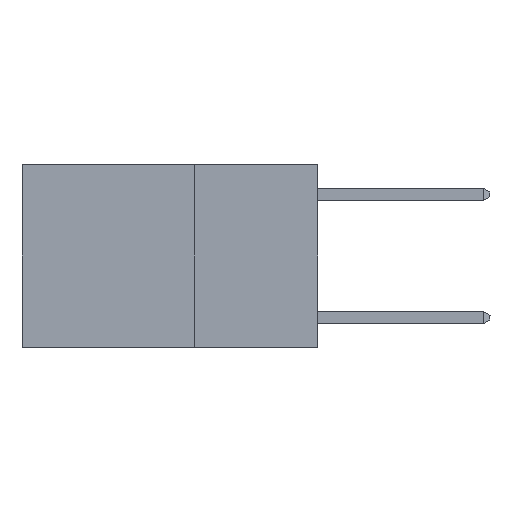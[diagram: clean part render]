
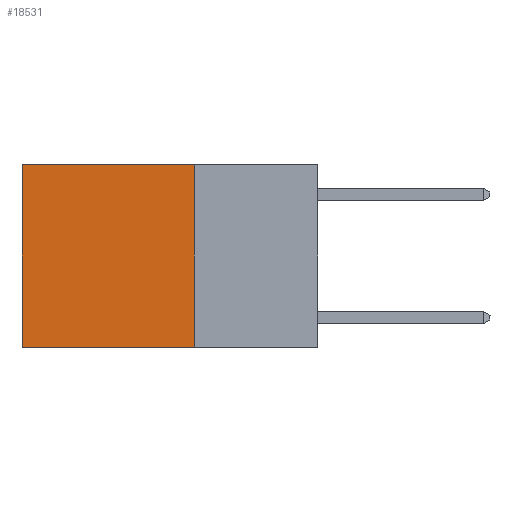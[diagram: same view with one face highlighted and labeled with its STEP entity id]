
A CAD part, left-side view. The second image highlights one B-rep face of the part: STEP entity #18531.
In plain terms, the highlighted planar face has unit normal (-1, 0, 0).
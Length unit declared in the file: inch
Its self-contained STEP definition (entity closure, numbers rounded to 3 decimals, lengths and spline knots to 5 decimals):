
#1092 = DIRECTION ( 'NONE',  ( 0., 0., -1. ) ) ;
#1262 = DIRECTION ( 'NONE',  ( 1., 0., 0. ) ) ;
#1551 = VECTOR ( 'NONE', #5936, 39.37008 ) ;
#1714 = VECTOR ( 'NONE', #1092, 39.37008 ) ;
#1950 = CARTESIAN_POINT ( 'NONE',  ( 0.2625, 0.25, 0. ) ) ;
#2614 = VERTEX_POINT ( 'NONE', #6307 ) ;
#3176 = EDGE_CURVE ( 'NONE', #8763, #2614, #7273, .T. ) ;
#3692 = VECTOR ( 'NONE', #7816, 39.37008 ) ;
#4391 = CARTESIAN_POINT ( 'NONE',  ( 0.2625, 0.25, -0.37 ) ) ;
#5743 = LINE ( 'NONE', #7167, #1714 ) ;
#5936 = DIRECTION ( 'NONE',  ( 0., 0., -1. ) ) ;
#6307 = CARTESIAN_POINT ( 'NONE',  ( 0.2625, 0.6, -0.37 ) ) ;
#7167 = CARTESIAN_POINT ( 'NONE',  ( 0.2625, 0.25, 0. ) ) ;
#7273 = LINE ( 'NONE', #18326, #3692 ) ;
#7395 = CARTESIAN_POINT ( 'NONE',  ( 0.2625, 0.6, 0. ) ) ;
#7660 = EDGE_CURVE ( 'NONE', #11700, #14391, #18274, .T. ) ;
#7816 = DIRECTION ( 'NONE',  ( 0., 1., 0. ) ) ;
#8507 = VECTOR ( 'NONE', #9395, 39.37008 ) ;
#8763 = VERTEX_POINT ( 'NONE', #4391 ) ;
#9139 = LINE ( 'NONE', #19642, #1551 ) ;
#9267 = CARTESIAN_POINT ( 'NONE',  ( 0.2625, 0.25, 0. ) ) ;
#9395 = DIRECTION ( 'NONE',  ( 0., 1., 0. ) ) ;
#11389 = ORIENTED_EDGE ( 'NONE', *, *, #15072, .F. ) ;
#11700 = VERTEX_POINT ( 'NONE', #1950 ) ;
#11852 = FACE_OUTER_BOUND ( 'NONE', #15990, .T. ) ;
#12399 = ORIENTED_EDGE ( 'NONE', *, *, #7660, .T. ) ;
#13516 = EDGE_CURVE ( 'NONE', #14391, #2614, #9139, .T. ) ;
#13574 = ORIENTED_EDGE ( 'NONE', *, *, #13516, .T. ) ;
#14391 = VERTEX_POINT ( 'NONE', #7395 ) ;
#14800 = PLANE ( 'NONE',  #19624 ) ;
#15072 = EDGE_CURVE ( 'NONE', #11700, #8763, #5743, .T. ) ;
#15990 = EDGE_LOOP ( 'NONE', ( #13574, #18620, #11389, #12399 ) ) ;
#16313 = CARTESIAN_POINT ( 'NONE',  ( 0.2625, 0.25, 0. ) ) ;
#16515 = DIRECTION ( 'NONE',  ( 0., 0., -1. ) ) ;
#18274 = LINE ( 'NONE', #9267, #8507 ) ;
#18326 = CARTESIAN_POINT ( 'NONE',  ( 0.2625, 0.25, -0.37 ) ) ;
#18531 = ADVANCED_FACE ( 'NONE', ( #11852 ), #14800, .F. ) ;
#18620 = ORIENTED_EDGE ( 'NONE', *, *, #3176, .F. ) ;
#19624 = AXIS2_PLACEMENT_3D ( 'NONE', #16313, #1262, #16515 ) ;
#19642 = CARTESIAN_POINT ( 'NONE',  ( 0.2625, 0.6, 0. ) ) ;
